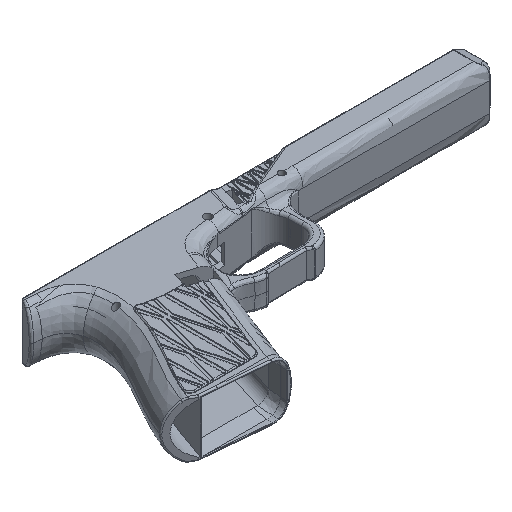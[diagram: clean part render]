
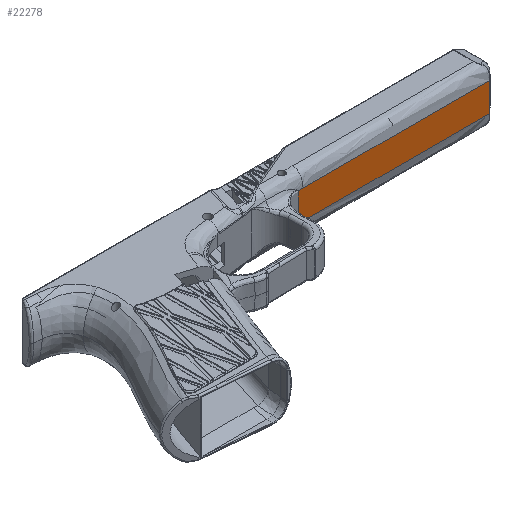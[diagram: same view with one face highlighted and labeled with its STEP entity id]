
A CAD part, isometric view. The second image highlights one B-rep face of the part: STEP entity #22278.
In plain terms, the highlighted planar face has unit normal (0, -1, 0).
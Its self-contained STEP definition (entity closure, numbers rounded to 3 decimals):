
#1126=PLANE('',#23623);
#1884=LINE('',#29700,#3755);
#1961=LINE('',#31475,#3832);
#1962=LINE('',#31482,#3833);
#1963=LINE('',#31488,#3834);
#3755=VECTOR('',#24687,10.);
#3832=VECTOR('',#24864,10.);
#3833=VECTOR('',#24865,1.);
#3834=VECTOR('',#24866,10.);
#5664=B_SPLINE_CURVE_WITH_KNOTS('',3,(#31477,#31478,#31479,#31480),
 .UNSPECIFIED.,.F.,.F.,(4,4),(0.,0.277),.UNSPECIFIED.);
#5665=B_SPLINE_CURVE_WITH_KNOTS('',3,(#31484,#31485,#31486,#31487),
 .UNSPECIFIED.,.F.,.F.,(4,4),(0.,0.277),.UNSPECIFIED.);
#6516=FACE_OUTER_BOUND('',#7822,.T.);
#7822=EDGE_LOOP('',(#15454,#15455,#15456,#15457,#15458,#15459));
#9424=VERTEX_POINT('',#29692);
#9425=VERTEX_POINT('',#29699);
#9517=VERTEX_POINT('',#31474);
#9518=VERTEX_POINT('',#31476);
#9519=VERTEX_POINT('',#31481);
#9520=VERTEX_POINT('',#31483);
#11679=EDGE_CURVE('',#9424,#9425,#1884,.T.);
#11805=EDGE_CURVE('',#9517,#9424,#1961,.T.);
#11806=EDGE_CURVE('',#9518,#9517,#5664,.T.);
#11807=EDGE_CURVE('',#9519,#9518,#1962,.T.);
#11808=EDGE_CURVE('',#9519,#9520,#5665,.T.);
#11809=EDGE_CURVE('',#9520,#9425,#1963,.T.);
#15454=ORIENTED_EDGE('',*,*,#11805,.F.);
#15455=ORIENTED_EDGE('',*,*,#11806,.F.);
#15456=ORIENTED_EDGE('',*,*,#11807,.F.);
#15457=ORIENTED_EDGE('',*,*,#11808,.T.);
#15458=ORIENTED_EDGE('',*,*,#11809,.T.);
#15459=ORIENTED_EDGE('',*,*,#11679,.F.);
#22278=ADVANCED_FACE('',(#6516),#1126,.T.);
#23623=AXIS2_PLACEMENT_3D('',#31473,#24862,#24863);
#24687=DIRECTION('',(0.,0.,-1.));
#24862=DIRECTION('center_axis',(0.,-1.,0.));
#24863=DIRECTION('ref_axis',(1.,0.,0.));
#24864=DIRECTION('',(1.,0.,0.));
#24865=DIRECTION('',(0.,0.,1.));
#24866=DIRECTION('',(1.,0.,0.));
#29692=CARTESIAN_POINT('',(220.785,-17.,7.246));
#29699=CARTESIAN_POINT('',(220.785,-17.,-7.246));
#29700=CARTESIAN_POINT('',(220.785,-17.,-14.4));
#31473=CARTESIAN_POINT('Origin',(103.503,-17.,-14.4));
#31474=CARTESIAN_POINT('',(126.,-17.,7.246));
#31475=CARTESIAN_POINT('',(126.,-17.,7.246));
#31476=CARTESIAN_POINT('',(123.81,-17.,7.237));
#31477=CARTESIAN_POINT('Ctrl Pts',(123.81,-17.,7.237));
#31478=CARTESIAN_POINT('Ctrl Pts',(124.54,-17.,7.24));
#31479=CARTESIAN_POINT('Ctrl Pts',(125.27,-17.,7.243));
#31480=CARTESIAN_POINT('Ctrl Pts',(126.,-17.,7.246));
#31481=CARTESIAN_POINT('',(123.81,-17.,-7.237));
#31482=CARTESIAN_POINT('',(123.81,-17.,-7.237));
#31483=CARTESIAN_POINT('',(126.,-17.,-7.246));
#31484=CARTESIAN_POINT('Ctrl Pts',(123.81,-17.,-7.237));
#31485=CARTESIAN_POINT('Ctrl Pts',(124.54,-17.,-7.24));
#31486=CARTESIAN_POINT('Ctrl Pts',(125.27,-17.,-7.243));
#31487=CARTESIAN_POINT('Ctrl Pts',(126.,-17.,-7.246));
#31488=CARTESIAN_POINT('',(126.,-17.,-7.246));
